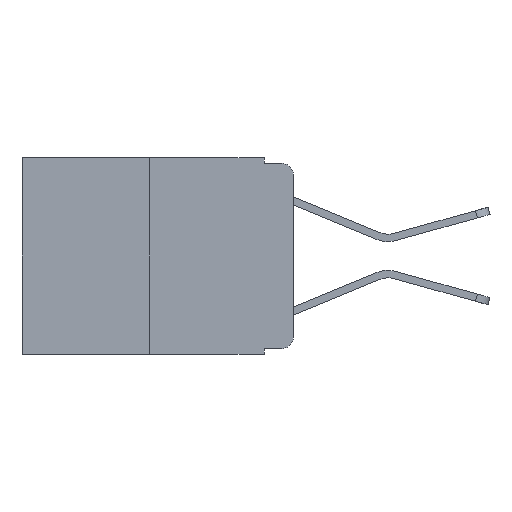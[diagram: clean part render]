
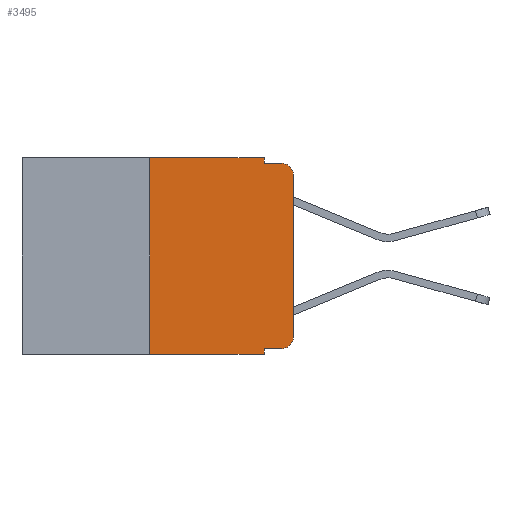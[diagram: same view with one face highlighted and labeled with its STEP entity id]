
A CAD part, left-side view. The second image highlights one B-rep face of the part: STEP entity #3495.
In plain terms, the highlighted planar face has unit normal (-1, 0, 0).
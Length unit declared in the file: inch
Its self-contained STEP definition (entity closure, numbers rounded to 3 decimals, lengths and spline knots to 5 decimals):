
#171 = EDGE_CURVE ( 'NONE', #2910, #4093, #3177, .T. ) ;
#207 = CARTESIAN_POINT ( 'NONE',  ( 0., 0., -0.313 ) ) ;
#670 = CARTESIAN_POINT ( 'NONE',  ( 0., 0., 0. ) ) ;
#829 = CARTESIAN_POINT ( 'NONE',  ( 0., 0.473, 0. ) ) ;
#944 = EDGE_CURVE ( 'NONE', #11489, #11050, #9404, .T. ) ;
#1013 = CARTESIAN_POINT ( 'NONE',  ( 0., 0.473, -0.343 ) ) ;
#1027 = EDGE_CURVE ( 'NONE', #3041, #1636, #11255, .T. ) ;
#1029 = AXIS2_PLACEMENT_3D ( 'NONE', #2328, #5418, #6012 ) ;
#1215 = DIRECTION ( 'NONE',  ( -1., 0., 0. ) ) ;
#1296 = CIRCLE ( 'NONE', #10985, 0.02 ) ;
#1371 = VECTOR ( 'NONE', #11273, 39.37008 ) ;
#1469 = VECTOR ( 'NONE', #9182, 39.37008 ) ;
#1520 = VERTEX_POINT ( 'NONE', #3307 ) ;
#1636 = VERTEX_POINT ( 'NONE', #207 ) ;
#1719 = EDGE_CURVE ( 'NONE', #12564, #3041, #10684, .T. ) ;
#1879 = PLANE ( 'NONE',  #8261 ) ;
#2328 = CARTESIAN_POINT ( 'NONE',  ( 0., 0.02, -0.313 ) ) ;
#2898 = CARTESIAN_POINT ( 'NONE',  ( 0., 0.051, -0.333 ) ) ;
#2910 = VERTEX_POINT ( 'NONE', #12317 ) ;
#2976 = VECTOR ( 'NONE', #12157, 39.37008 ) ;
#3014 = CARTESIAN_POINT ( 'NONE',  ( 0., 0.02, -0.01 ) ) ;
#3041 = VERTEX_POINT ( 'NONE', #5942 ) ;
#3177 = LINE ( 'NONE', #6434, #10576 ) ;
#3307 = CARTESIAN_POINT ( 'NONE',  ( 0., 0.051, -0.01 ) ) ;
#3314 = ORIENTED_EDGE ( 'NONE', *, *, #1027, .T. ) ;
#3367 = ORIENTED_EDGE ( 'NONE', *, *, #1719, .T. ) ;
#3495 = ADVANCED_FACE ( 'NONE', ( #5377 ), #1879, .F. ) ;
#3684 = ORIENTED_EDGE ( 'NONE', *, *, #3937, .F. ) ;
#3937 = EDGE_CURVE ( 'NONE', #12564, #11050, #9266, .T. ) ;
#4093 = VERTEX_POINT ( 'NONE', #5054 ) ;
#4152 = ORIENTED_EDGE ( 'NONE', *, *, #944, .T. ) ;
#4153 = VECTOR ( 'NONE', #11109, 39.37008 ) ;
#4274 = LINE ( 'NONE', #5757, #1371 ) ;
#4282 = DIRECTION ( 'NONE',  ( 0., 0., -1. ) ) ;
#4549 = CARTESIAN_POINT ( 'NONE',  ( 0., 0.051, 0. ) ) ;
#4808 = CARTESIAN_POINT ( 'NONE',  ( 0., 0.051, -0.333 ) ) ;
#5054 = CARTESIAN_POINT ( 'NONE',  ( 0., 0.051, 0. ) ) ;
#5339 = DIRECTION ( 'NONE',  ( 0., 0., -1. ) ) ;
#5377 = FACE_OUTER_BOUND ( 'NONE', #9309, .T. ) ;
#5418 = DIRECTION ( 'NONE',  ( -1., 0., 0. ) ) ;
#5568 = CARTESIAN_POINT ( 'NONE',  ( 0., 0.051, -0.343 ) ) ;
#5757 = CARTESIAN_POINT ( 'NONE',  ( 0., 0.051, -0.01 ) ) ;
#5942 = CARTESIAN_POINT ( 'NONE',  ( 0., 0.02, -0.333 ) ) ;
#5993 = EDGE_CURVE ( 'NONE', #11489, #2910, #11898, .T. ) ;
#6012 = DIRECTION ( 'NONE',  ( 0., 0., -1. ) ) ;
#6073 = DIRECTION ( 'NONE',  ( 0., -1., 0. ) ) ;
#6434 = CARTESIAN_POINT ( 'NONE',  ( 0., 0.473, 0. ) ) ;
#6615 = EDGE_CURVE ( 'NONE', #4093, #1520, #11058, .T. ) ;
#6827 = VECTOR ( 'NONE', #11080, 39.37008 ) ;
#7177 = ORIENTED_EDGE ( 'NONE', *, *, #5993, .F. ) ;
#7341 = VERTEX_POINT ( 'NONE', #3014 ) ;
#7362 = CARTESIAN_POINT ( 'NONE',  ( 0., 0.02, -0.03 ) ) ;
#7443 = ORIENTED_EDGE ( 'NONE', *, *, #171, .F. ) ;
#7849 = EDGE_CURVE ( 'NONE', #1520, #7341, #4274, .T. ) ;
#7939 = VERTEX_POINT ( 'NONE', #11334 ) ;
#8261 = AXIS2_PLACEMENT_3D ( 'NONE', #829, #9958, #4282 ) ;
#8281 = DIRECTION ( 'NONE',  ( 0., 0., -1. ) ) ;
#8345 = CARTESIAN_POINT ( 'NONE',  ( 0., 0.25, 0. ) ) ;
#8369 = LINE ( 'NONE', #670, #10529 ) ;
#8454 = EDGE_CURVE ( 'NONE', #7939, #7341, #1296, .T. ) ;
#8720 = DIRECTION ( 'NONE',  ( 0., 0., 1. ) ) ;
#9182 = DIRECTION ( 'NONE',  ( 0., -1., 0. ) ) ;
#9266 = LINE ( 'NONE', #4549, #6827 ) ;
#9309 = EDGE_LOOP ( 'NONE', ( #10747, #11294, #12603, #11209, #7443, #7177, #4152, #3684, #3367, #3314 ) ) ;
#9404 = LINE ( 'NONE', #1013, #1469 ) ;
#9700 = EDGE_CURVE ( 'NONE', #1636, #7939, #8369, .T. ) ;
#9728 = CARTESIAN_POINT ( 'NONE',  ( 0., 0.25, -0.343 ) ) ;
#9958 = DIRECTION ( 'NONE',  ( 1., 0., 0. ) ) ;
#10529 = VECTOR ( 'NONE', #8720, 39.37008 ) ;
#10576 = VECTOR ( 'NONE', #6073, 39.37008 ) ;
#10684 = LINE ( 'NONE', #4808, #2976 ) ;
#10747 = ORIENTED_EDGE ( 'NONE', *, *, #9700, .T. ) ;
#10771 = VECTOR ( 'NONE', #5339, 39.37008 ) ;
#10853 = CARTESIAN_POINT ( 'NONE',  ( 0., 0.051, 0. ) ) ;
#10985 = AXIS2_PLACEMENT_3D ( 'NONE', #7362, #1215, #8281 ) ;
#11050 = VERTEX_POINT ( 'NONE', #5568 ) ;
#11058 = LINE ( 'NONE', #10853, #10771 ) ;
#11080 = DIRECTION ( 'NONE',  ( 0., 0., -1. ) ) ;
#11109 = DIRECTION ( 'NONE',  ( 0., 0., 1. ) ) ;
#11209 = ORIENTED_EDGE ( 'NONE', *, *, #6615, .F. ) ;
#11255 = CIRCLE ( 'NONE', #1029, 0.02 ) ;
#11273 = DIRECTION ( 'NONE',  ( 0., -1., 0. ) ) ;
#11294 = ORIENTED_EDGE ( 'NONE', *, *, #8454, .T. ) ;
#11334 = CARTESIAN_POINT ( 'NONE',  ( 0., 0., -0.03 ) ) ;
#11489 = VERTEX_POINT ( 'NONE', #9728 ) ;
#11898 = LINE ( 'NONE', #8345, #4153 ) ;
#12157 = DIRECTION ( 'NONE',  ( 0., -1., 0. ) ) ;
#12317 = CARTESIAN_POINT ( 'NONE',  ( 0., 0.25, 0. ) ) ;
#12564 = VERTEX_POINT ( 'NONE', #2898 ) ;
#12603 = ORIENTED_EDGE ( 'NONE', *, *, #7849, .F. ) ;
